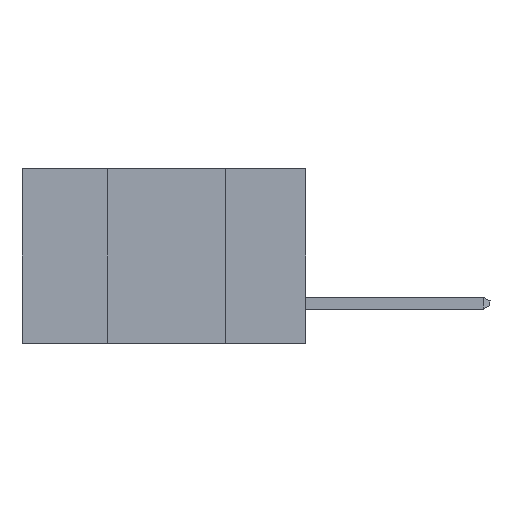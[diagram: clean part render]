
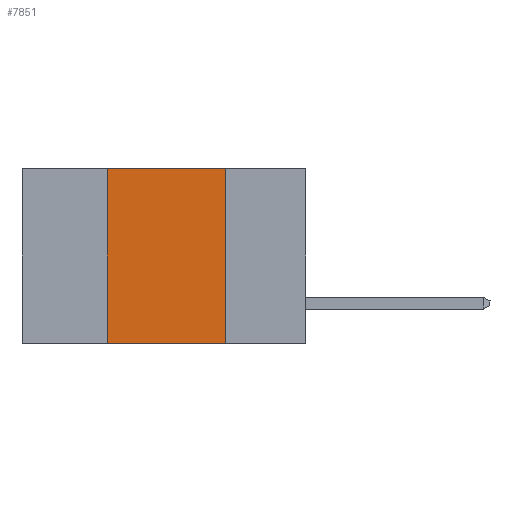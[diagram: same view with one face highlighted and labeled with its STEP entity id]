
A CAD part, left-side view. The second image highlights one B-rep face of the part: STEP entity #7851.
In plain terms, the highlighted planar face has unit normal (-1, 0, 0).
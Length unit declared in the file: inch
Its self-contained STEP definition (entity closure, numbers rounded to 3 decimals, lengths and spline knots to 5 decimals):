
#286 = DIRECTION ( 'NONE',  ( 0., 0., -1. ) ) ;
#388 = CARTESIAN_POINT ( 'NONE',  ( 0., 0.6, 0. ) ) ;
#571 = LINE ( 'NONE', #388, #16809 ) ;
#1043 = CARTESIAN_POINT ( 'NONE',  ( 0., 0.42, -0.37 ) ) ;
#1870 = LINE ( 'NONE', #4615, #11788 ) ;
#2156 = CARTESIAN_POINT ( 'NONE',  ( 0., 0.17, -0.37 ) ) ;
#2250 = CARTESIAN_POINT ( 'NONE',  ( 0., 0.17, 0. ) ) ;
#2319 = EDGE_CURVE ( 'NONE', #4058, #7834, #8654, .T. ) ;
#3055 = VERTEX_POINT ( 'NONE', #2156 ) ;
#3129 = DIRECTION ( 'NONE',  ( 0., -1., 0. ) ) ;
#3833 = PLANE ( 'NONE',  #7042 ) ;
#3975 = CARTESIAN_POINT ( 'NONE',  ( 0., 0.6, -0.37 ) ) ;
#4058 = VERTEX_POINT ( 'NONE', #1043 ) ;
#4615 = CARTESIAN_POINT ( 'NONE',  ( 0., 0.17, -0.37 ) ) ;
#5336 = EDGE_LOOP ( 'NONE', ( #9788, #11073, #15723, #7938 ) ) ;
#5669 = VECTOR ( 'NONE', #6271, 39.37008 ) ;
#6099 = VERTEX_POINT ( 'NONE', #2250 ) ;
#6271 = DIRECTION ( 'NONE',  ( 0., 0., 1. ) ) ;
#6380 = CARTESIAN_POINT ( 'NONE',  ( 0., 0.6, 0. ) ) ;
#6468 = EDGE_CURVE ( 'NONE', #7834, #6099, #571, .T. ) ;
#6563 = FACE_OUTER_BOUND ( 'NONE', #5336, .T. ) ;
#6753 = EDGE_CURVE ( 'NONE', #6099, #3055, #1870, .T. ) ;
#7042 = AXIS2_PLACEMENT_3D ( 'NONE', #6380, #11668, #10518 ) ;
#7834 = VERTEX_POINT ( 'NONE', #13258 ) ;
#7851 = ADVANCED_FACE ( 'NONE', ( #6563 ), #3833, .F. ) ;
#7938 = ORIENTED_EDGE ( 'NONE', *, *, #12098, .T. ) ;
#8654 = LINE ( 'NONE', #14353, #5669 ) ;
#9788 = ORIENTED_EDGE ( 'NONE', *, *, #6753, .F. ) ;
#10518 = DIRECTION ( 'NONE',  ( 0., 0., -1. ) ) ;
#11073 = ORIENTED_EDGE ( 'NONE', *, *, #6468, .F. ) ;
#11668 = DIRECTION ( 'NONE',  ( 1., 0., 0. ) ) ;
#11788 = VECTOR ( 'NONE', #286, 39.37008 ) ;
#12098 = EDGE_CURVE ( 'NONE', #4058, #3055, #13232, .T. ) ;
#13232 = LINE ( 'NONE', #3975, #14958 ) ;
#13258 = CARTESIAN_POINT ( 'NONE',  ( 0., 0.42, 0. ) ) ;
#14353 = CARTESIAN_POINT ( 'NONE',  ( 0., 0.42, -0.37 ) ) ;
#14958 = VECTOR ( 'NONE', #16191, 39.37008 ) ;
#15723 = ORIENTED_EDGE ( 'NONE', *, *, #2319, .F. ) ;
#16191 = DIRECTION ( 'NONE',  ( 0., -1., 0. ) ) ;
#16809 = VECTOR ( 'NONE', #3129, 39.37008 ) ;
